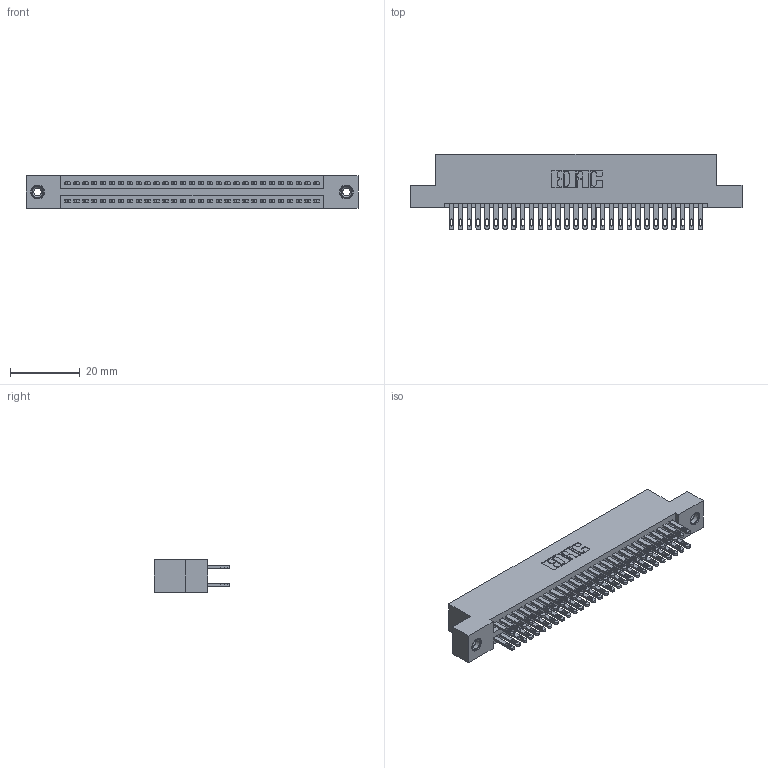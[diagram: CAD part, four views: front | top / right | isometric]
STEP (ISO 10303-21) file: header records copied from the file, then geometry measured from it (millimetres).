
FILE_DESCRIPTION (( 'STEP AP203' ), '1' );
FILE_NAME ('345-058-500-208.STEP', '2018-09-19T04:05:43', ( '' ), ( '' ), 'SwSTEP 2.0', 'SolidWorks 2016', '' );
FILE_SCHEMA (( 'CONFIG_CONTROL_DESIGN' ));
Length unit declared in the file: inch
Products named in the file (4): 345-058-500-208; 345 Part_Flush Mounting Lugs - 0.156 Dia-TI; 345-292-001_345-293-100; 345-250-001_345-250-003-102
Assembly tree (61 placements, depth 2):
  345-058-500-208
    345 Part_Flush Mounting Lugs - 0.156 Dia-TI
    345-292-001_345-293-100  x58
    345-250-001_345-250-003-102  x2
Bounding box: 94.87 x 21.51 x 9.4 mm (x, y, z)
Volume: 9265.7 mm3; surface area: 14049.5 mm2
Topology: 61 solids, 61 shells, 2854 faces, 8655 edges, 5762 vertices
Faces by surface type: plane 1678, cylinder 1160, cone 12, torus 4
Entity records: 25620 total; most frequent: CARTESIAN_POINT 4287, ORIENTED_EDGE 4214, DIRECTION 3825, EDGE_CURVE 2107, LINE 1835, VECTOR 1835, VERTEX_POINT 1400, AXIS2_PLACEMENT_3D 995
